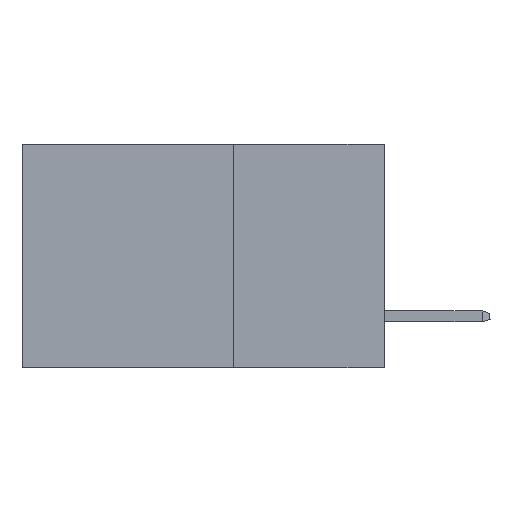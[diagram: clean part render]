
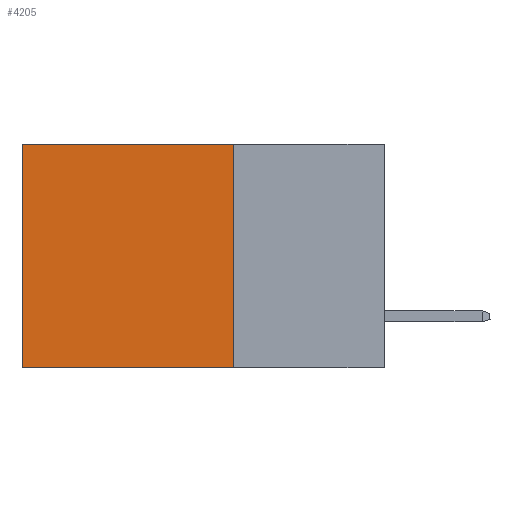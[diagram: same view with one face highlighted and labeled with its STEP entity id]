
A CAD part, left-side view. The second image highlights one B-rep face of the part: STEP entity #4205.
In plain terms, the highlighted planar face has unit normal (-1, 0, 0).
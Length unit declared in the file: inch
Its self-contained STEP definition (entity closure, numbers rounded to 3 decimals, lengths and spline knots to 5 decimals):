
#658 = DIRECTION ( 'NONE',  ( 0., 0., -1. ) ) ;
#1004 = VERTEX_POINT ( 'NONE', #12024 ) ;
#1450 = CARTESIAN_POINT ( 'NONE',  ( 0.2615, 0.6, 0. ) ) ;
#1529 = LINE ( 'NONE', #5431, #12989 ) ;
#2034 = PLANE ( 'NONE',  #6472 ) ;
#2722 = EDGE_CURVE ( 'NONE', #12724, #12776, #1529, .T. ) ;
#2848 = DIRECTION ( 'NONE',  ( 0., 1., 0. ) ) ;
#3161 = DIRECTION ( 'NONE',  ( 0., 0., -1. ) ) ;
#3205 = EDGE_CURVE ( 'NONE', #14223, #1004, #5256, .T. ) ;
#3842 = CARTESIAN_POINT ( 'NONE',  ( 0.2615, 0.25, 0. ) ) ;
#4205 = ADVANCED_FACE ( 'NONE', ( #5930 ), #2034, .F. ) ;
#4590 = EDGE_CURVE ( 'NONE', #12776, #1004, #12563, .T. ) ;
#5256 = LINE ( 'NONE', #9014, #7425 ) ;
#5431 = CARTESIAN_POINT ( 'NONE',  ( 0.2615, 0.25, -0.37 ) ) ;
#5930 = FACE_OUTER_BOUND ( 'NONE', #6893, .T. ) ;
#6472 = AXIS2_PLACEMENT_3D ( 'NONE', #12738, #6646, #11388 ) ;
#6646 = DIRECTION ( 'NONE',  ( 1., 0., 0. ) ) ;
#6893 = EDGE_LOOP ( 'NONE', ( #10670, #8753, #12213, #11982 ) ) ;
#7425 = VECTOR ( 'NONE', #3161, 39.37008 ) ;
#8336 = DIRECTION ( 'NONE',  ( 0., 1., 0. ) ) ;
#8753 = ORIENTED_EDGE ( 'NONE', *, *, #4590, .F. ) ;
#9014 = CARTESIAN_POINT ( 'NONE',  ( 0.2615, 0.6, -0.37 ) ) ;
#9146 = LINE ( 'NONE', #3842, #9905 ) ;
#9667 = CARTESIAN_POINT ( 'NONE',  ( 0.2615, 0.25, -0.37 ) ) ;
#9905 = VECTOR ( 'NONE', #8336, 39.37008 ) ;
#10670 = ORIENTED_EDGE ( 'NONE', *, *, #3205, .T. ) ;
#10718 = VECTOR ( 'NONE', #2848, 39.37008 ) ;
#11039 = CARTESIAN_POINT ( 'NONE',  ( 0.2615, 0.25, -0.37 ) ) ;
#11388 = DIRECTION ( 'NONE',  ( 0., 0., -1. ) ) ;
#11982 = ORIENTED_EDGE ( 'NONE', *, *, #14185, .T. ) ;
#12024 = CARTESIAN_POINT ( 'NONE',  ( 0.2615, 0.6, -0.37 ) ) ;
#12213 = ORIENTED_EDGE ( 'NONE', *, *, #2722, .F. ) ;
#12563 = LINE ( 'NONE', #11039, #10718 ) ;
#12724 = VERTEX_POINT ( 'NONE', #14323 ) ;
#12738 = CARTESIAN_POINT ( 'NONE',  ( 0.2615, 0.25, -0.37 ) ) ;
#12776 = VERTEX_POINT ( 'NONE', #9667 ) ;
#12989 = VECTOR ( 'NONE', #658, 39.37008 ) ;
#14185 = EDGE_CURVE ( 'NONE', #12724, #14223, #9146, .T. ) ;
#14223 = VERTEX_POINT ( 'NONE', #1450 ) ;
#14323 = CARTESIAN_POINT ( 'NONE',  ( 0.2615, 0.25, 0. ) ) ;
